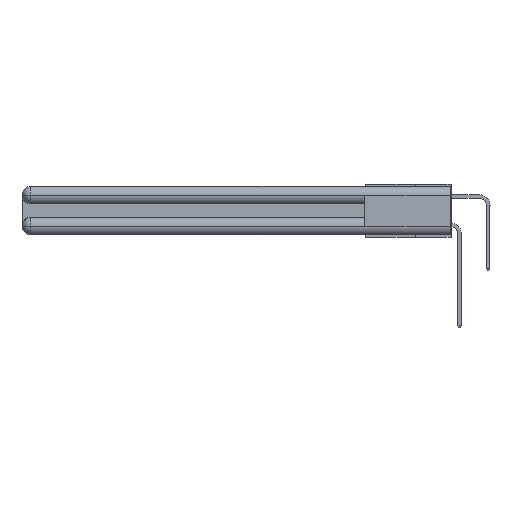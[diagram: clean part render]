
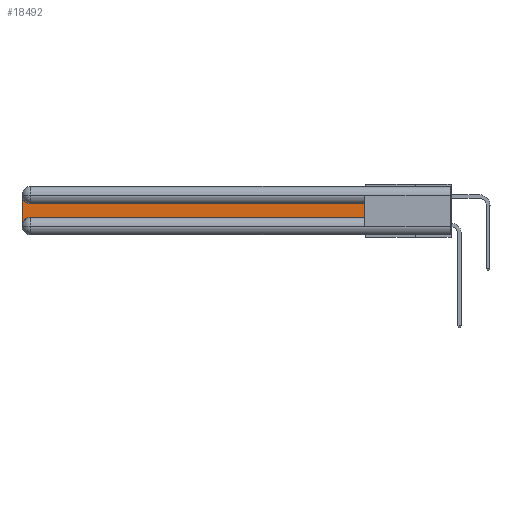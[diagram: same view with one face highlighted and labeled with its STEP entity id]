
A CAD part, left-side view. The second image highlights one B-rep face of the part: STEP entity #18492.
In plain terms, the highlighted planar face has unit normal (-1, 0, 0).
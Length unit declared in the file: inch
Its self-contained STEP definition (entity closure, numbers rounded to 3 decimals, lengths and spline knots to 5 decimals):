
#1260 = AXIS2_PLACEMENT_3D ( 'NONE', #19946, #17403, #11903 ) ;
#1444 = ORIENTED_EDGE ( 'NONE', *, *, #25677, .T. ) ;
#1552 = LINE ( 'NONE', #23608, #4443 ) ;
#1880 = CARTESIAN_POINT ( 'NONE',  ( 0.075, 2.94, -0.1225 ) ) ;
#2982 = DIRECTION ( 'NONE',  ( 0., 1., 0. ) ) ;
#4443 = VECTOR ( 'NONE', #21035, 39.37008 ) ;
#5636 = DIRECTION ( 'NONE',  ( 0., 0., -1. ) ) ;
#6240 = ORIENTED_EDGE ( 'NONE', *, *, #6251, .T. ) ;
#6251 = EDGE_CURVE ( 'NONE', #12928, #21842, #16273, .T. ) ;
#6292 = VECTOR ( 'NONE', #7198, 39.37008 ) ;
#6835 = DIRECTION ( 'NONE',  ( 0., 0., 1. ) ) ;
#7198 = DIRECTION ( 'NONE',  ( 0., 0., -1. ) ) ;
#9639 = ORIENTED_EDGE ( 'NONE', *, *, #30300, .T. ) ;
#9973 = CARTESIAN_POINT ( 'NONE',  ( 0.075, 3., -0.2175 ) ) ;
#10377 = EDGE_CURVE ( 'NONE', #26773, #26048, #31209, .T. ) ;
#11792 = VECTOR ( 'NONE', #2982, 39.37008 ) ;
#11903 = DIRECTION ( 'NONE',  ( 0., 0., -1. ) ) ;
#12842 = DIRECTION ( 'NONE',  ( 1., 0., 0. ) ) ;
#12928 = VERTEX_POINT ( 'NONE', #1880 ) ;
#13697 = DIRECTION ( 'NONE',  ( 1., 0., 0. ) ) ;
#13850 = CARTESIAN_POINT ( 'NONE',  ( 0.075, 0.6, -0.2175 ) ) ;
#13915 = CARTESIAN_POINT ( 'NONE',  ( 0.075, 2.94, -0.0625 ) ) ;
#15759 = AXIS2_PLACEMENT_3D ( 'NONE', #13915, #13697, #5636 ) ;
#16173 = CARTESIAN_POINT ( 'NONE',  ( 0.075, 0.6, -0.1225 ) ) ;
#16273 = CIRCLE ( 'NONE', #15759, 0.06 ) ;
#16395 = LINE ( 'NONE', #16173, #11792 ) ;
#16801 = ORIENTED_EDGE ( 'NONE', *, *, #23198, .T. ) ;
#16842 = FACE_OUTER_BOUND ( 'NONE', #29353, .T. ) ;
#16908 = CARTESIAN_POINT ( 'NONE',  ( 0.075, 0.6, -0.2175 ) ) ;
#17403 = DIRECTION ( 'NONE',  ( 1., 0., 0. ) ) ;
#18492 = ADVANCED_FACE ( 'NONE', ( #16842 ), #30877, .F. ) ;
#19143 = VERTEX_POINT ( 'NONE', #20488 ) ;
#19946 = CARTESIAN_POINT ( 'NONE',  ( 0.075, 2.94, -0.2775 ) ) ;
#20025 = LINE ( 'NONE', #9973, #6292 ) ;
#20488 = CARTESIAN_POINT ( 'NONE',  ( 0.075, 3., -0.2775 ) ) ;
#20783 = VECTOR ( 'NONE', #6835, 39.37008 ) ;
#21035 = DIRECTION ( 'NONE',  ( 0., -1., 0. ) ) ;
#21529 = ORIENTED_EDGE ( 'NONE', *, *, #28379, .T. ) ;
#21842 = VERTEX_POINT ( 'NONE', #30786 ) ;
#22312 = CIRCLE ( 'NONE', #1260, 0.06 ) ;
#22967 = CARTESIAN_POINT ( 'NONE',  ( 0.075, 3., -0.1225 ) ) ;
#23029 = AXIS2_PLACEMENT_3D ( 'NONE', #22967, #12842, #29691 ) ;
#23198 = EDGE_CURVE ( 'NONE', #19143, #30015, #22312, .T. ) ;
#23608 = CARTESIAN_POINT ( 'NONE',  ( 0.075, 0.6, -0.2175 ) ) ;
#25677 = EDGE_CURVE ( 'NONE', #21842, #19143, #20025, .T. ) ;
#26048 = VERTEX_POINT ( 'NONE', #32622 ) ;
#26773 = VERTEX_POINT ( 'NONE', #16908 ) ;
#28379 = EDGE_CURVE ( 'NONE', #30015, #26773, #1552, .T. ) ;
#29353 = EDGE_LOOP ( 'NONE', ( #9639, #6240, #1444, #16801, #21529, #31145 ) ) ;
#29691 = DIRECTION ( 'NONE',  ( 0., 0., -1. ) ) ;
#30015 = VERTEX_POINT ( 'NONE', #34153 ) ;
#30300 = EDGE_CURVE ( 'NONE', #26048, #12928, #16395, .T. ) ;
#30786 = CARTESIAN_POINT ( 'NONE',  ( 0.075, 3., -0.0625 ) ) ;
#30877 = PLANE ( 'NONE',  #23029 ) ;
#31145 = ORIENTED_EDGE ( 'NONE', *, *, #10377, .T. ) ;
#31209 = LINE ( 'NONE', #13850, #20783 ) ;
#32622 = CARTESIAN_POINT ( 'NONE',  ( 0.075, 0.6, -0.1225 ) ) ;
#34153 = CARTESIAN_POINT ( 'NONE',  ( 0.075, 2.94, -0.2175 ) ) ;
